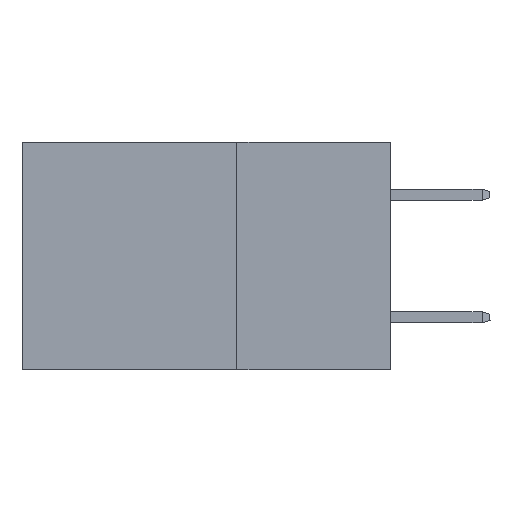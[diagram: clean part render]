
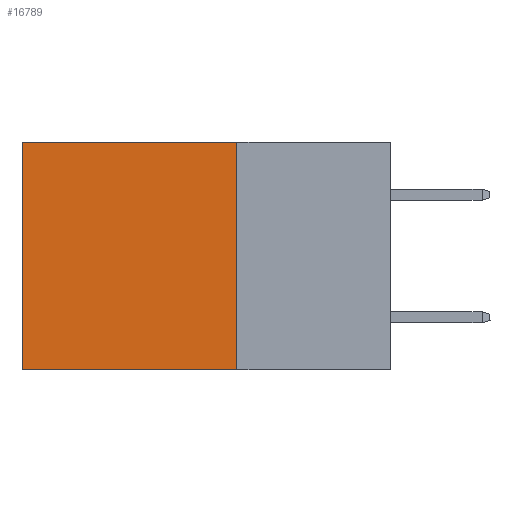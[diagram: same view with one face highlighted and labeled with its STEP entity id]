
A CAD part, left-side view. The second image highlights one B-rep face of the part: STEP entity #16789.
In plain terms, the highlighted planar face has unit normal (-1, 0, 0).
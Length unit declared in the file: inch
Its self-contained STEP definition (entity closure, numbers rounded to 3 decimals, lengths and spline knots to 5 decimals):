
#832 = PLANE ( 'NONE',  #1943 ) ;
#1943 = AXIS2_PLACEMENT_3D ( 'NONE', #4636, #16525, #2699 ) ;
#2148 = VERTEX_POINT ( 'NONE', #2706 ) ;
#2374 = DIRECTION ( 'NONE',  ( 0., 1., 0. ) ) ;
#2699 = DIRECTION ( 'NONE',  ( 0., 0., -1. ) ) ;
#2706 = CARTESIAN_POINT ( 'NONE',  ( 0.2875, 0.25, 0. ) ) ;
#2879 = LINE ( 'NONE', #11331, #25164 ) ;
#2921 = EDGE_CURVE ( 'NONE', #2148, #14088, #23051, .T. ) ;
#3087 = CARTESIAN_POINT ( 'NONE',  ( 0.2875, 0.25, -0.37 ) ) ;
#3541 = DIRECTION ( 'NONE',  ( 0., 0., -1. ) ) ;
#3555 = EDGE_CURVE ( 'NONE', #2148, #11734, #2879, .T. ) ;
#3973 = CARTESIAN_POINT ( 'NONE',  ( 0.2875, 0.6, 0. ) ) ;
#4071 = CARTESIAN_POINT ( 'NONE',  ( 0.2875, 0.25, -0.37 ) ) ;
#4125 = DIRECTION ( 'NONE',  ( 0., 1., 0. ) ) ;
#4140 = CARTESIAN_POINT ( 'NONE',  ( 0.2875, 0.6, 0. ) ) ;
#4158 = ORIENTED_EDGE ( 'NONE', *, *, #2921, .T. ) ;
#4636 = CARTESIAN_POINT ( 'NONE',  ( 0.2875, 0.25, 0. ) ) ;
#4941 = FACE_OUTER_BOUND ( 'NONE', #25165, .T. ) ;
#5348 = VECTOR ( 'NONE', #4125, 39.37008 ) ;
#6782 = ORIENTED_EDGE ( 'NONE', *, *, #9351, .F. ) ;
#7528 = ORIENTED_EDGE ( 'NONE', *, *, #3555, .F. ) ;
#7836 = CARTESIAN_POINT ( 'NONE',  ( 0.2875, 0.6, -0.37 ) ) ;
#9351 = EDGE_CURVE ( 'NONE', #11734, #16534, #16865, .T. ) ;
#9791 = EDGE_CURVE ( 'NONE', #14088, #16534, #16843, .T. ) ;
#11331 = CARTESIAN_POINT ( 'NONE',  ( 0.2875, 0.25, 0. ) ) ;
#11734 = VERTEX_POINT ( 'NONE', #3087 ) ;
#14088 = VERTEX_POINT ( 'NONE', #4140 ) ;
#15669 = ORIENTED_EDGE ( 'NONE', *, *, #9791, .T. ) ;
#16017 = CARTESIAN_POINT ( 'NONE',  ( 0.2875, 0.25, 0. ) ) ;
#16525 = DIRECTION ( 'NONE',  ( 1., 0., 0. ) ) ;
#16534 = VERTEX_POINT ( 'NONE', #7836 ) ;
#16789 = ADVANCED_FACE ( 'NONE', ( #4941 ), #832, .F. ) ;
#16843 = LINE ( 'NONE', #3973, #22616 ) ;
#16865 = LINE ( 'NONE', #4071, #22640 ) ;
#17666 = DIRECTION ( 'NONE',  ( 0., 0., -1. ) ) ;
#22616 = VECTOR ( 'NONE', #17666, 39.37008 ) ;
#22640 = VECTOR ( 'NONE', #2374, 39.37008 ) ;
#23051 = LINE ( 'NONE', #16017, #5348 ) ;
#25164 = VECTOR ( 'NONE', #3541, 39.37008 ) ;
#25165 = EDGE_LOOP ( 'NONE', ( #15669, #6782, #7528, #4158 ) ) ;
